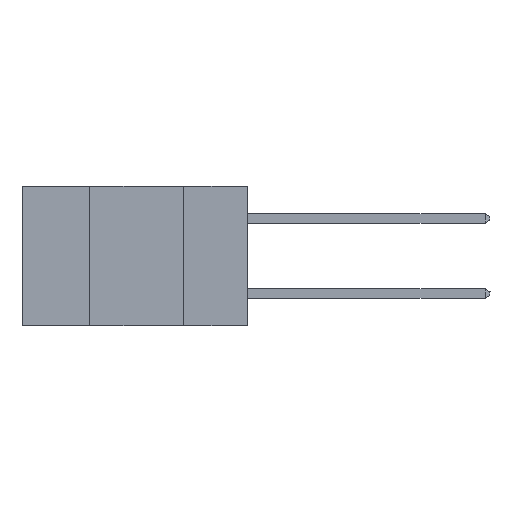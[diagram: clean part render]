
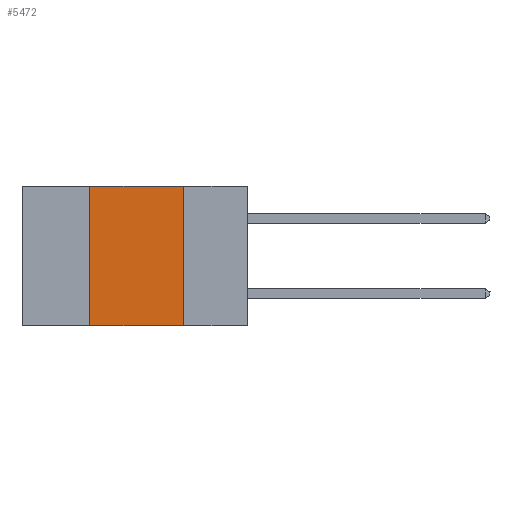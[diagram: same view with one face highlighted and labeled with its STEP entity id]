
A CAD part, left-side view. The second image highlights one B-rep face of the part: STEP entity #5472.
In plain terms, the highlighted planar face has unit normal (-1, 0, 0).
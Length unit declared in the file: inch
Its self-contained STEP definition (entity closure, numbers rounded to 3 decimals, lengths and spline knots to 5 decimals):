
#934 = VERTEX_POINT ( 'NONE', #4382 ) ;
#1212 = ORIENTED_EDGE ( 'NONE', *, *, #12496, .F. ) ;
#1270 = LINE ( 'NONE', #5891, #20439 ) ;
#1531 = CARTESIAN_POINT ( 'NONE',  ( 0., 0.17, -0.37 ) ) ;
#1614 = ORIENTED_EDGE ( 'NONE', *, *, #5433, .F. ) ;
#4177 = EDGE_LOOP ( 'NONE', ( #1212, #13584, #1614, #8670 ) ) ;
#4221 = VECTOR ( 'NONE', #6795, 39.37008 ) ;
#4382 = CARTESIAN_POINT ( 'NONE',  ( 0., 0.42, -0.37 ) ) ;
#4525 = LINE ( 'NONE', #24595, #19151 ) ;
#4997 = AXIS2_PLACEMENT_3D ( 'NONE', #7781, #20929, #9703 ) ;
#5433 = EDGE_CURVE ( 'NONE', #934, #14345, #4525, .T. ) ;
#5472 = ADVANCED_FACE ( 'NONE', ( #8517 ), #17226, .F. ) ;
#5891 = CARTESIAN_POINT ( 'NONE',  ( 0., 0.17, -0.37 ) ) ;
#6720 = VECTOR ( 'NONE', #20103, 39.37008 ) ;
#6795 = DIRECTION ( 'NONE',  ( 0., -1., 0. ) ) ;
#7781 = CARTESIAN_POINT ( 'NONE',  ( 0., 0.6, 0. ) ) ;
#8517 = FACE_OUTER_BOUND ( 'NONE', #4177, .T. ) ;
#8670 = ORIENTED_EDGE ( 'NONE', *, *, #23876, .T. ) ;
#9426 = CARTESIAN_POINT ( 'NONE',  ( 0., 0.17, 0. ) ) ;
#9703 = DIRECTION ( 'NONE',  ( 0., 0., -1. ) ) ;
#12496 = EDGE_CURVE ( 'NONE', #17117, #22767, #1270, .T. ) ;
#12616 = CARTESIAN_POINT ( 'NONE',  ( 0., 0.6, -0.37 ) ) ;
#13584 = ORIENTED_EDGE ( 'NONE', *, *, #15469, .F. ) ;
#14345 = VERTEX_POINT ( 'NONE', #22573 ) ;
#15445 = DIRECTION ( 'NONE',  ( 0., 0., -1. ) ) ;
#15469 = EDGE_CURVE ( 'NONE', #14345, #17117, #18273, .T. ) ;
#16852 = LINE ( 'NONE', #12616, #6720 ) ;
#17117 = VERTEX_POINT ( 'NONE', #9426 ) ;
#17149 = DIRECTION ( 'NONE',  ( 0., 0., 1. ) ) ;
#17226 = PLANE ( 'NONE',  #4997 ) ;
#18273 = LINE ( 'NONE', #23702, #4221 ) ;
#19151 = VECTOR ( 'NONE', #17149, 39.37008 ) ;
#20103 = DIRECTION ( 'NONE',  ( 0., -1., 0. ) ) ;
#20439 = VECTOR ( 'NONE', #15445, 39.37008 ) ;
#20929 = DIRECTION ( 'NONE',  ( 1., 0., 0. ) ) ;
#22573 = CARTESIAN_POINT ( 'NONE',  ( 0., 0.42, 0. ) ) ;
#22767 = VERTEX_POINT ( 'NONE', #1531 ) ;
#23702 = CARTESIAN_POINT ( 'NONE',  ( 0., 0.6, 0. ) ) ;
#23876 = EDGE_CURVE ( 'NONE', #934, #22767, #16852, .T. ) ;
#24595 = CARTESIAN_POINT ( 'NONE',  ( 0., 0.42, -0.37 ) ) ;
